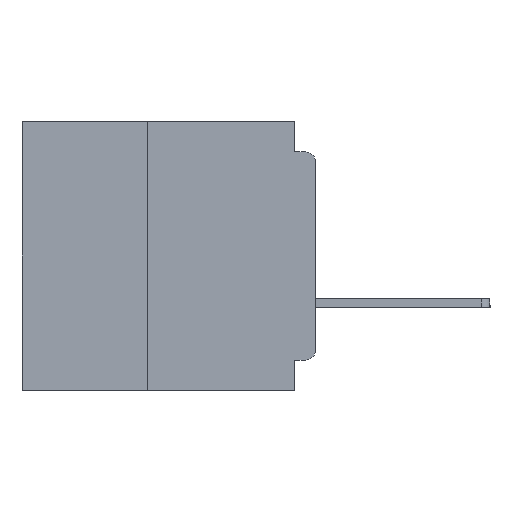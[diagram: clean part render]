
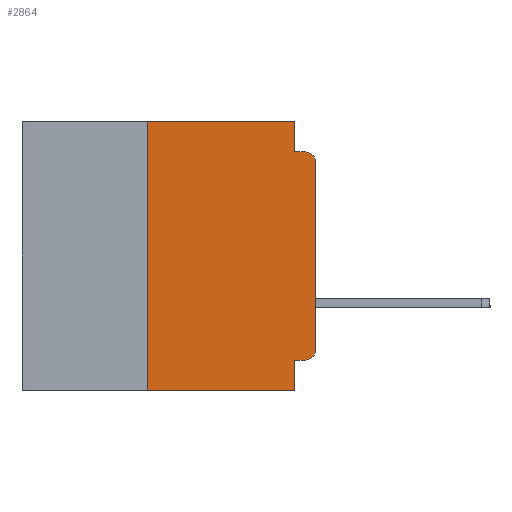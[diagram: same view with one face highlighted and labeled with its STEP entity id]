
A CAD part, left-side view. The second image highlights one B-rep face of the part: STEP entity #2864.
In plain terms, the highlighted planar face has unit normal (-1, 0, 0).
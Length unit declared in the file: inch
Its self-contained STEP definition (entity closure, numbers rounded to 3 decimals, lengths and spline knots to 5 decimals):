
#439 = CARTESIAN_POINT ( 'NONE',  ( 0., 0., -0.045 ) ) ;
#530 = DIRECTION ( 'NONE',  ( 0., 0., -1. ) ) ;
#1162 = VECTOR ( 'NONE', #22667, 39.37008 ) ;
#2421 = AXIS2_PLACEMENT_3D ( 'NONE', #20944, #25021, #530 ) ;
#2864 = ADVANCED_FACE ( 'NONE', ( #46171 ), #45171, .F. ) ;
#3034 = ORIENTED_EDGE ( 'NONE', *, *, #3237, .T. ) ;
#3237 = EDGE_CURVE ( 'NONE', #35676, #19798, #51183, .T. ) ;
#3869 = ORIENTED_EDGE ( 'NONE', *, *, #45271, .F. ) ;
#4023 = DIRECTION ( 'NONE',  ( -1., 0., 0. ) ) ;
#5125 = EDGE_CURVE ( 'NONE', #50438, #21008, #10226, .T. ) ;
#5824 = CARTESIAN_POINT ( 'NONE',  ( 0., 0.015, -0.045 ) ) ;
#5868 = ORIENTED_EDGE ( 'NONE', *, *, #7089, .F. ) ;
#6129 = CARTESIAN_POINT ( 'NONE',  ( 0., 0.031, -0.4 ) ) ;
#7089 = EDGE_CURVE ( 'NONE', #21008, #34028, #29599, .T. ) ;
#7095 = ORIENTED_EDGE ( 'NONE', *, *, #39827, .F. ) ;
#8689 = DIRECTION ( 'NONE',  ( 0., 0., 1. ) ) ;
#9688 = VECTOR ( 'NONE', #52392, 39.37008 ) ;
#10226 = LINE ( 'NONE', #15742, #20966 ) ;
#10647 = CARTESIAN_POINT ( 'NONE',  ( 0., 0., 0. ) ) ;
#10879 = CARTESIAN_POINT ( 'NONE',  ( 0., 0., -0.355 ) ) ;
#10974 = LINE ( 'NONE', #20040, #9688 ) ;
#11353 = ORIENTED_EDGE ( 'NONE', *, *, #32305, .T. ) ;
#12243 = EDGE_LOOP ( 'NONE', ( #11353, #13828, #5868, #37477, #7095, #19662, #3034, #3869, #30067, #25495 ) ) ;
#12741 = DIRECTION ( 'NONE',  ( 0., -1., 0. ) ) ;
#12762 = VERTEX_POINT ( 'NONE', #30365 ) ;
#13151 = LINE ( 'NONE', #20746, #44129 ) ;
#13558 = CIRCLE ( 'NONE', #29272, 0.015 ) ;
#13828 = ORIENTED_EDGE ( 'NONE', *, *, #26111, .T. ) ;
#14879 = CARTESIAN_POINT ( 'NONE',  ( 0., 0.25, -0.4 ) ) ;
#15409 = CARTESIAN_POINT ( 'NONE',  ( 0., 0.015, -0.06 ) ) ;
#15742 = CARTESIAN_POINT ( 'NONE',  ( 0., 0.031, 0. ) ) ;
#18855 = EDGE_CURVE ( 'NONE', #34273, #12762, #13558, .T. ) ;
#18862 = VECTOR ( 'NONE', #12741, 39.37008 ) ;
#19025 = DIRECTION ( 'NONE',  ( 0., 1., 0. ) ) ;
#19319 = CARTESIAN_POINT ( 'NONE',  ( 0., 0.437, -0.4 ) ) ;
#19443 = LINE ( 'NONE', #6129, #28931 ) ;
#19473 = DIRECTION ( 'NONE',  ( 0., 0., -1. ) ) ;
#19662 = ORIENTED_EDGE ( 'NONE', *, *, #51080, .F. ) ;
#19798 = VERTEX_POINT ( 'NONE', #46697 ) ;
#20040 = CARTESIAN_POINT ( 'NONE',  ( 0., 0.437, 0. ) ) ;
#20154 = VERTEX_POINT ( 'NONE', #40808 ) ;
#20746 = CARTESIAN_POINT ( 'NONE',  ( 0., 0.25, -0.4 ) ) ;
#20944 = CARTESIAN_POINT ( 'NONE',  ( 0., 0.437, 0. ) ) ;
#20966 = VECTOR ( 'NONE', #27756, 39.37008 ) ;
#21008 = VERTEX_POINT ( 'NONE', #30295 ) ;
#22667 = DIRECTION ( 'NONE',  ( 0., 0., 1. ) ) ;
#22887 = LINE ( 'NONE', #10647, #1162 ) ;
#24426 = CIRCLE ( 'NONE', #27489, 0.015 ) ;
#24540 = CARTESIAN_POINT ( 'NONE',  ( 0., 0.031, 0. ) ) ;
#25021 = DIRECTION ( 'NONE',  ( 1., 0., 0. ) ) ;
#25495 = ORIENTED_EDGE ( 'NONE', *, *, #18855, .T. ) ;
#26111 = EDGE_CURVE ( 'NONE', #47873, #34028, #24426, .T. ) ;
#27489 = AXIS2_PLACEMENT_3D ( 'NONE', #15409, #43681, #19473 ) ;
#27576 = LINE ( 'NONE', #10879, #47830 ) ;
#27756 = DIRECTION ( 'NONE',  ( 0., 0., -1. ) ) ;
#28416 = CARTESIAN_POINT ( 'NONE',  ( 0., 0.015, -0.34 ) ) ;
#28931 = VECTOR ( 'NONE', #38565, 39.37008 ) ;
#29272 = AXIS2_PLACEMENT_3D ( 'NONE', #28416, #4023, #32454 ) ;
#29599 = LINE ( 'NONE', #439, #18862 ) ;
#30067 = ORIENTED_EDGE ( 'NONE', *, *, #46531, .F. ) ;
#30295 = CARTESIAN_POINT ( 'NONE',  ( 0., 0.031, -0.045 ) ) ;
#30365 = CARTESIAN_POINT ( 'NONE',  ( 0., 0., -0.34 ) ) ;
#31703 = CARTESIAN_POINT ( 'NONE',  ( 0., 0.015, -0.355 ) ) ;
#32305 = EDGE_CURVE ( 'NONE', #12762, #47873, #22887, .T. ) ;
#32454 = DIRECTION ( 'NONE',  ( 0., 0., -1. ) ) ;
#34028 = VERTEX_POINT ( 'NONE', #5824 ) ;
#34273 = VERTEX_POINT ( 'NONE', #31703 ) ;
#35676 = VERTEX_POINT ( 'NONE', #14879 ) ;
#37195 = CARTESIAN_POINT ( 'NONE',  ( 0., 0.031, -0.355 ) ) ;
#37477 = ORIENTED_EDGE ( 'NONE', *, *, #5125, .F. ) ;
#38565 = DIRECTION ( 'NONE',  ( 0., 0., -1. ) ) ;
#39827 = EDGE_CURVE ( 'NONE', #20154, #50438, #10974, .T. ) ;
#40808 = CARTESIAN_POINT ( 'NONE',  ( 0., 0.25, 0. ) ) ;
#41666 = VECTOR ( 'NONE', #47611, 39.37008 ) ;
#43138 = CARTESIAN_POINT ( 'NONE',  ( 0., 0., -0.06 ) ) ;
#43681 = DIRECTION ( 'NONE',  ( -1., 0., 0. ) ) ;
#44129 = VECTOR ( 'NONE', #8689, 39.37008 ) ;
#45171 = PLANE ( 'NONE',  #2421 ) ;
#45271 = EDGE_CURVE ( 'NONE', #48860, #19798, #19443, .T. ) ;
#46171 = FACE_OUTER_BOUND ( 'NONE', #12243, .T. ) ;
#46531 = EDGE_CURVE ( 'NONE', #34273, #48860, #27576, .T. ) ;
#46697 = CARTESIAN_POINT ( 'NONE',  ( 0., 0.031, -0.4 ) ) ;
#47611 = DIRECTION ( 'NONE',  ( 0., -1., 0. ) ) ;
#47830 = VECTOR ( 'NONE', #19025, 39.37008 ) ;
#47873 = VERTEX_POINT ( 'NONE', #43138 ) ;
#48860 = VERTEX_POINT ( 'NONE', #37195 ) ;
#50438 = VERTEX_POINT ( 'NONE', #24540 ) ;
#51080 = EDGE_CURVE ( 'NONE', #35676, #20154, #13151, .T. ) ;
#51183 = LINE ( 'NONE', #19319, #41666 ) ;
#52392 = DIRECTION ( 'NONE',  ( 0., -1., 0. ) ) ;
